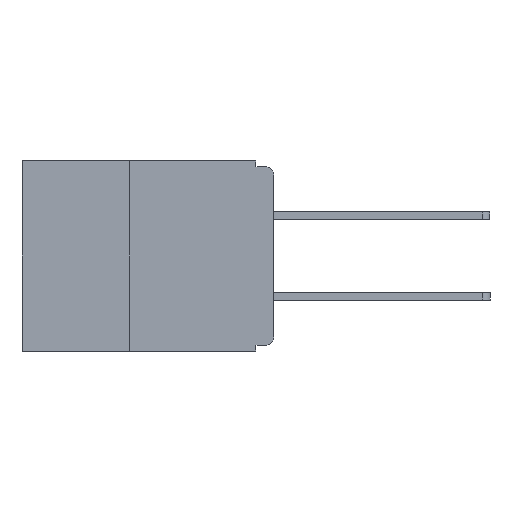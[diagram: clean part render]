
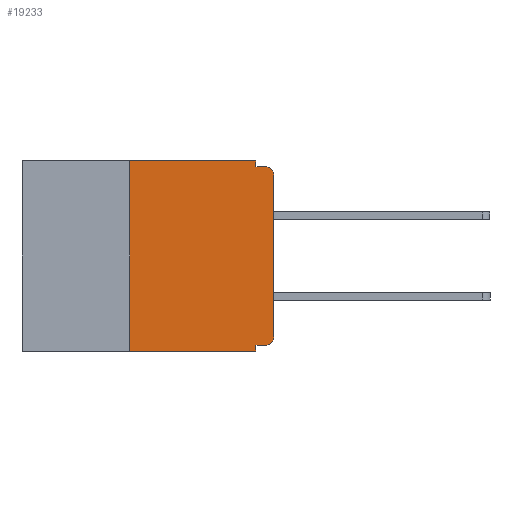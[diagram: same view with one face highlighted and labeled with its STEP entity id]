
A CAD part, left-side view. The second image highlights one B-rep face of the part: STEP entity #19233.
In plain terms, the highlighted planar face has unit normal (-1, 0, 0).
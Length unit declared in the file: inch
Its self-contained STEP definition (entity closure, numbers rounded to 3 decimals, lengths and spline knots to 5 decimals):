
#1207 = DIRECTION ( 'NONE',  ( 0., -1., 0. ) ) ;
#1308 = EDGE_CURVE ( 'NONE', #7171, #5275, #14344, .T. ) ;
#1514 = CARTESIAN_POINT ( 'NONE',  ( 0., 0., -0.01 ) ) ;
#1909 = CARTESIAN_POINT ( 'NONE',  ( 0., 0.015, -0.305 ) ) ;
#2729 = VECTOR ( 'NONE', #14645, 39.37008 ) ;
#2856 = VERTEX_POINT ( 'NONE', #11761 ) ;
#2950 = CARTESIAN_POINT ( 'NONE',  ( 0., 0.031, -0.32 ) ) ;
#3002 = ORIENTED_EDGE ( 'NONE', *, *, #21342, .F. ) ;
#3407 = EDGE_CURVE ( 'NONE', #9605, #17279, #10840, .T. ) ;
#3680 = CARTESIAN_POINT ( 'NONE',  ( 0., 0.031, -0.33 ) ) ;
#3685 = VECTOR ( 'NONE', #1207, 39.37008 ) ;
#3726 = CARTESIAN_POINT ( 'NONE',  ( 0., 0., 0. ) ) ;
#3957 = EDGE_CURVE ( 'NONE', #2856, #8864, #8320, .T. ) ;
#4107 = DIRECTION ( 'NONE',  ( 0., 0., -1. ) ) ;
#4211 = VERTEX_POINT ( 'NONE', #6226 ) ;
#4407 = AXIS2_PLACEMENT_3D ( 'NONE', #1909, #16228, #4107 ) ;
#4781 = VECTOR ( 'NONE', #11899, 39.37008 ) ;
#5126 = CARTESIAN_POINT ( 'NONE',  ( 0., 0.437, 0. ) ) ;
#5275 = VERTEX_POINT ( 'NONE', #14465 ) ;
#6226 = CARTESIAN_POINT ( 'NONE',  ( 0., 0.015, -0.01 ) ) ;
#6402 = CARTESIAN_POINT ( 'NONE',  ( 0., 0.25, 0. ) ) ;
#6672 = DIRECTION ( 'NONE',  ( -1., 0., 0. ) ) ;
#6984 = VERTEX_POINT ( 'NONE', #16678 ) ;
#7171 = VERTEX_POINT ( 'NONE', #2950 ) ;
#7227 = DIRECTION ( 'NONE',  ( 1., 0., 0. ) ) ;
#7418 = VECTOR ( 'NONE', #21819, 39.37008 ) ;
#7503 = DIRECTION ( 'NONE',  ( 0., 0., -1. ) ) ;
#7888 = VECTOR ( 'NONE', #23353, 39.37008 ) ;
#8320 = LINE ( 'NONE', #15016, #2729 ) ;
#8479 = EDGE_LOOP ( 'NONE', ( #17782, #10589, #18402, #9267, #14022, #8991, #25268, #22526, #3002, #19691 ) ) ;
#8619 = AXIS2_PLACEMENT_3D ( 'NONE', #18725, #6672, #20677 ) ;
#8864 = VERTEX_POINT ( 'NONE', #6402 ) ;
#8991 = ORIENTED_EDGE ( 'NONE', *, *, #3957, .F. ) ;
#9267 = ORIENTED_EDGE ( 'NONE', *, *, #3407, .F. ) ;
#9358 = CARTESIAN_POINT ( 'NONE',  ( 0., 0.015, -0.32 ) ) ;
#9605 = VERTEX_POINT ( 'NONE', #23242 ) ;
#9796 = FACE_OUTER_BOUND ( 'NONE', #8479, .T. ) ;
#10589 = ORIENTED_EDGE ( 'NONE', *, *, #10714, .T. ) ;
#10714 = EDGE_CURVE ( 'NONE', #18459, #4211, #20013, .T. ) ;
#10840 = LINE ( 'NONE', #13165, #4781 ) ;
#11368 = CARTESIAN_POINT ( 'NONE',  ( 0., 0.437, -0.33 ) ) ;
#11761 = CARTESIAN_POINT ( 'NONE',  ( 0., 0.25, -0.33 ) ) ;
#11899 = DIRECTION ( 'NONE',  ( 0., 0., -1. ) ) ;
#12257 = EDGE_CURVE ( 'NONE', #17279, #4211, #23936, .T. ) ;
#13165 = CARTESIAN_POINT ( 'NONE',  ( 0., 0.031, 0. ) ) ;
#14022 = ORIENTED_EDGE ( 'NONE', *, *, #18847, .F. ) ;
#14344 = LINE ( 'NONE', #3680, #19583 ) ;
#14374 = VECTOR ( 'NONE', #16361, 39.37008 ) ;
#14465 = CARTESIAN_POINT ( 'NONE',  ( 0., 0.031, -0.33 ) ) ;
#14540 = LINE ( 'NONE', #17617, #3685 ) ;
#14645 = DIRECTION ( 'NONE',  ( 0., 0., 1. ) ) ;
#15016 = CARTESIAN_POINT ( 'NONE',  ( 0., 0.25, -0.33 ) ) ;
#15793 = CIRCLE ( 'NONE', #4407, 0.015 ) ;
#16228 = DIRECTION ( 'NONE',  ( -1., 0., 0. ) ) ;
#16361 = DIRECTION ( 'NONE',  ( 0., 1., 0. ) ) ;
#16678 = CARTESIAN_POINT ( 'NONE',  ( 0., 0., -0.305 ) ) ;
#17244 = PLANE ( 'NONE',  #24826 ) ;
#17279 = VERTEX_POINT ( 'NONE', #24276 ) ;
#17617 = CARTESIAN_POINT ( 'NONE',  ( 0., 0.437, 0. ) ) ;
#17782 = ORIENTED_EDGE ( 'NONE', *, *, #20060, .T. ) ;
#18358 = CARTESIAN_POINT ( 'NONE',  ( 0., 0., -0.32 ) ) ;
#18391 = EDGE_CURVE ( 'NONE', #24238, #6984, #15793, .T. ) ;
#18402 = ORIENTED_EDGE ( 'NONE', *, *, #12257, .F. ) ;
#18459 = VERTEX_POINT ( 'NONE', #20185 ) ;
#18725 = CARTESIAN_POINT ( 'NONE',  ( 0., 0.015, -0.025 ) ) ;
#18847 = EDGE_CURVE ( 'NONE', #8864, #9605, #14540, .T. ) ;
#19233 = ADVANCED_FACE ( 'NONE', ( #9796 ), #17244, .F. ) ;
#19273 = EDGE_CURVE ( 'NONE', #2856, #5275, #23749, .T. ) ;
#19583 = VECTOR ( 'NONE', #7503, 39.37008 ) ;
#19691 = ORIENTED_EDGE ( 'NONE', *, *, #18391, .T. ) ;
#19693 = VECTOR ( 'NONE', #21835, 39.37008 ) ;
#20013 = CIRCLE ( 'NONE', #8619, 0.015 ) ;
#20060 = EDGE_CURVE ( 'NONE', #6984, #18459, #24916, .T. ) ;
#20185 = CARTESIAN_POINT ( 'NONE',  ( 0., 0., -0.025 ) ) ;
#20677 = DIRECTION ( 'NONE',  ( 0., 0., -1. ) ) ;
#21168 = DIRECTION ( 'NONE',  ( 0., 0., -1. ) ) ;
#21342 = EDGE_CURVE ( 'NONE', #24238, #7171, #24833, .T. ) ;
#21819 = DIRECTION ( 'NONE',  ( 0., -1., 0. ) ) ;
#21835 = DIRECTION ( 'NONE',  ( 0., 0., 1. ) ) ;
#22526 = ORIENTED_EDGE ( 'NONE', *, *, #1308, .F. ) ;
#23242 = CARTESIAN_POINT ( 'NONE',  ( 0., 0.031, 0. ) ) ;
#23353 = DIRECTION ( 'NONE',  ( 0., -1., 0. ) ) ;
#23749 = LINE ( 'NONE', #11368, #7888 ) ;
#23936 = LINE ( 'NONE', #1514, #7418 ) ;
#24238 = VERTEX_POINT ( 'NONE', #9358 ) ;
#24276 = CARTESIAN_POINT ( 'NONE',  ( 0., 0.031, -0.01 ) ) ;
#24826 = AXIS2_PLACEMENT_3D ( 'NONE', #5126, #7227, #21168 ) ;
#24833 = LINE ( 'NONE', #18358, #14374 ) ;
#24916 = LINE ( 'NONE', #3726, #19693 ) ;
#25268 = ORIENTED_EDGE ( 'NONE', *, *, #19273, .T. ) ;
